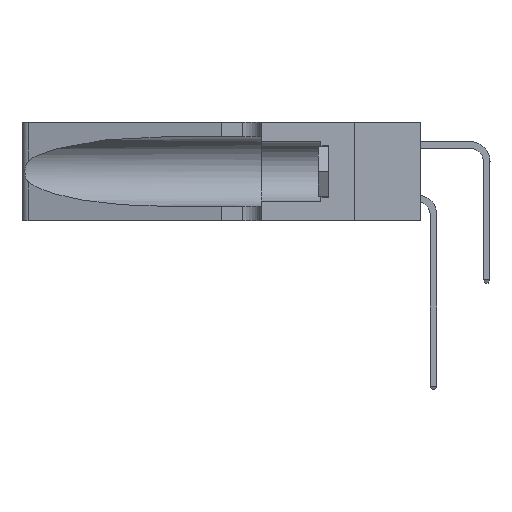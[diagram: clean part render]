
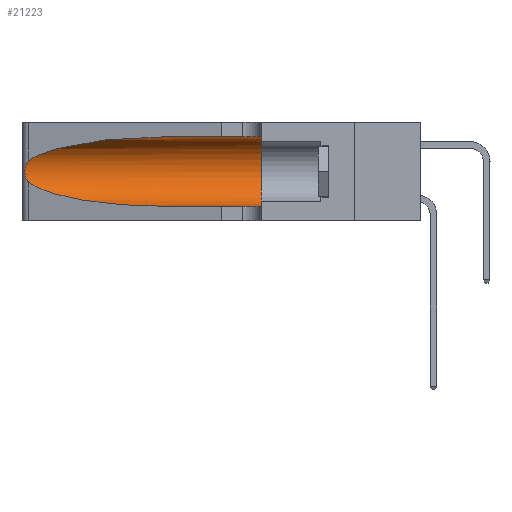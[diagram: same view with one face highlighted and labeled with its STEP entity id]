
A CAD part, left-side view. The second image highlights one B-rep face of the part: STEP entity #21223.
In plain terms, the highlighted cylindrical face has radius 3.308 mm (diameter 6.617 mm), a partial arc.
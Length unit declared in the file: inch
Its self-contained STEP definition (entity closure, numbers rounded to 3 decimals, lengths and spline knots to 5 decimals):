
#1243 = DIRECTION ( 'NONE',  ( 0., -1., 0. ) ) ;
#1526 = CARTESIAN_POINT ( 'NONE',  ( 0.25787, 1.23484, 0.2124 ) ) ;
#2860 = CARTESIAN_POINT ( 'NONE',  ( 0.1305, 0.72297, 0.31525 ) ) ;
#4259 = CARTESIAN_POINT ( 'NONE',  ( 0.1305, 0.35, 0.31525 ) ) ;
#4646 = CARTESIAN_POINT ( 'NONE',  ( 0.26018, 1.23835, 0.19895 ) ) ;
#5392 = EDGE_CURVE ( 'NONE', #9581, #30759, #23481, .T. ) ;
#5579 = CARTESIAN_POINT ( 'NONE',  ( 0.1305, 1.61858, 0.185 ) ) ;
#6573 = VERTEX_POINT ( 'NONE', #27221 ) ;
#7121 = CARTESIAN_POINT ( 'NONE',  ( 0.25487, 1.22718, 0.14631 ) ) ;
#7555 = CARTESIAN_POINT ( 'NONE',  ( 0.25555, 1.22994, 0.2215 ) ) ;
#7688 = CARTESIAN_POINT ( 'NONE',  ( 0.26075, 1.23896, 0.178 ) ) ;
#7708 = VERTEX_POINT ( 'NONE', #22228 ) ;
#7917 = CARTESIAN_POINT ( 'NONE',  ( 0.1305, 0.35, 0.185 ) ) ;
#8610 = DIRECTION ( 'NONE',  ( 0., -1., 0. ) ) ;
#8973 = CARTESIAN_POINT ( 'NONE',  ( 0.2373, 1.15595, 0.28018 ) ) ;
#9089 = B_SPLINE_CURVE_WITH_KNOTS ( 'NONE', 3,
 ( #30851, #7555, #19284, #1526, #22216, #4646, #25169, #7688, #28072, #10667, #30979, #32416, #15508, #35829 ),
 .UNSPECIFIED., .F., .F.,
 ( 4, 2, 2, 2, 2, 2, 4 ),
 ( 0., 0.00027, 0.00053, 0.00107, 0.0016, 0.00187, 0.00214 ),
 .UNSPECIFIED. ) ;
#9581 = VERTEX_POINT ( 'NONE', #4259 ) ;
#10316 = ORIENTED_EDGE ( 'NONE', *, *, #26908, .T. ) ;
#10667 = CARTESIAN_POINT ( 'NONE',  ( 0.25856, 1.23593, 0.16098 ) ) ;
#10898 = DIRECTION ( 'NONE',  ( 0., 0., 1. ) ) ;
#12828 = CARTESIAN_POINT ( 'NONE',  ( 0.25487, 1.22718, 0.14631 ) ) ;
#14348 = CARTESIAN_POINT ( 'NONE',  ( 0.1305, 0.35, 0.05475 ) ) ;
#14918 = AXIS2_PLACEMENT_3D ( 'NONE', #5579, #8610, #34681 ) ;
#15110 = CYLINDRICAL_SURFACE ( 'NONE', #14918, 0.13025 ) ;
#15508 = CARTESIAN_POINT ( 'NONE',  ( 0.25555, 1.22993, 0.14849 ) ) ;
#15738 = CARTESIAN_POINT ( 'NONE',  ( 0.18966, 0.96281, 0.05475 ) ) ;
#15906 = CARTESIAN_POINT ( 'NONE',  ( 0.1305, 0.72297, 0.05475 ) ) ;
#16090 = VECTOR ( 'NONE', #1243, 39.37008 ) ;
#16158 = ORIENTED_EDGE ( 'NONE', *, *, #35165, .T. ) ;
#16712 = VECTOR ( 'NONE', #34319, 39.37008 ) ;
#16898 = CARTESIAN_POINT ( 'NONE',  ( 0.1305, 1.61858, 0.31525 ) ) ;
#17850 = ORIENTED_EDGE ( 'NONE', *, *, #31130, .T. ) ;
#19284 = CARTESIAN_POINT ( 'NONE',  ( 0.25639, 1.23184, 0.21858 ) ) ;
#19825 =( BOUNDED_CURVE ( )  B_SPLINE_CURVE ( 3, ( #12828, #33141, #15738, #36064 ),
 .UNSPECIFIED., .F., .T. ) 
 B_SPLINE_CURVE_WITH_KNOTS ( ( 4, 4 ),
 ( 3.44316, 4.71239 ),
 .UNSPECIFIED. ) 
 CURVE ( )  GEOMETRIC_REPRESENTATION_ITEM ( )  RATIONAL_B_SPLINE_CURVE ( ( 1., 0.87, 0.87, 1. ) ) 
 REPRESENTATION_ITEM ( '' )  );
#20761 = ORIENTED_EDGE ( 'NONE', *, *, #28053, .F. ) ;
#21223 = ADVANCED_FACE ( 'NONE', ( #23777 ), #15110, .F. ) ;
#22216 = CARTESIAN_POINT ( 'NONE',  ( 0.25854, 1.2359, 0.20912 ) ) ;
#22228 = CARTESIAN_POINT ( 'NONE',  ( 0.25487, 1.22718, 0.22369 ) ) ;
#23481 = CIRCLE ( 'NONE', #37497, 0.13025 ) ;
#23777 = FACE_OUTER_BOUND ( 'NONE', #29883, .T. ) ;
#25169 = CARTESIAN_POINT ( 'NONE',  ( 0.26075, 1.23896, 0.19203 ) ) ;
#26908 = EDGE_CURVE ( 'NONE', #6573, #7708, #29371, .T. ) ;
#27221 = CARTESIAN_POINT ( 'NONE',  ( 0.1305, 0.72297, 0.31525 ) ) ;
#28053 = EDGE_CURVE ( 'NONE', #6573, #9581, #31285, .T. ) ;
#28072 = CARTESIAN_POINT ( 'NONE',  ( 0.26017, 1.23833, 0.17102 ) ) ;
#28297 = DIRECTION ( 'NONE',  ( 0., 1., 0. ) ) ;
#29313 = CARTESIAN_POINT ( 'NONE',  ( 0.25487, 1.22718, 0.22369 ) ) ;
#29371 =( BOUNDED_CURVE ( )  B_SPLINE_CURVE ( 3, ( #2860, #35034, #8973, #29313 ),
 .UNSPECIFIED., .F., .T. ) 
 B_SPLINE_CURVE_WITH_KNOTS ( ( 4, 4 ),
 ( 1.5708, 2.84003 ),
 .UNSPECIFIED. ) 
 CURVE ( )  GEOMETRIC_REPRESENTATION_ITEM ( )  RATIONAL_B_SPLINE_CURVE ( ( 1., 0.87, 0.87, 1. ) ) 
 REPRESENTATION_ITEM ( '' )  );
#29751 = VERTEX_POINT ( 'NONE', #7121 ) ;
#29883 = EDGE_LOOP ( 'NONE', ( #10316, #17850, #16158, #36177, #38050, #20761 ) ) ;
#30759 = VERTEX_POINT ( 'NONE', #14348 ) ;
#30851 = CARTESIAN_POINT ( 'NONE',  ( 0.25487, 1.22718, 0.22369 ) ) ;
#30979 = CARTESIAN_POINT ( 'NONE',  ( 0.25789, 1.23486, 0.15765 ) ) ;
#31130 = EDGE_CURVE ( 'NONE', #7708, #29751, #9089, .T. ) ;
#31285 = LINE ( 'NONE', #16898, #16712 ) ;
#31566 = LINE ( 'NONE', #36424, #16090 ) ;
#32416 = CARTESIAN_POINT ( 'NONE',  ( 0.25639, 1.23186, 0.15144 ) ) ;
#33141 = CARTESIAN_POINT ( 'NONE',  ( 0.2373, 1.15595, 0.08982 ) ) ;
#33816 = EDGE_CURVE ( 'NONE', #34568, #30759, #31566, .T. ) ;
#34319 = DIRECTION ( 'NONE',  ( 0., -1., 0. ) ) ;
#34568 = VERTEX_POINT ( 'NONE', #15906 ) ;
#34681 = DIRECTION ( 'NONE',  ( 0., 0., -1. ) ) ;
#35034 = CARTESIAN_POINT ( 'NONE',  ( 0.18966, 0.96281, 0.31525 ) ) ;
#35165 = EDGE_CURVE ( 'NONE', #29751, #34568, #19825, .T. ) ;
#35829 = CARTESIAN_POINT ( 'NONE',  ( 0.25487, 1.22718, 0.14631 ) ) ;
#36064 = CARTESIAN_POINT ( 'NONE',  ( 0.1305, 0.72297, 0.05475 ) ) ;
#36177 = ORIENTED_EDGE ( 'NONE', *, *, #33816, .T. ) ;
#36424 = CARTESIAN_POINT ( 'NONE',  ( 0.1305, 1.61858, 0.05475 ) ) ;
#37497 = AXIS2_PLACEMENT_3D ( 'NONE', #7917, #28297, #10898 ) ;
#38050 = ORIENTED_EDGE ( 'NONE', *, *, #5392, .F. ) ;
